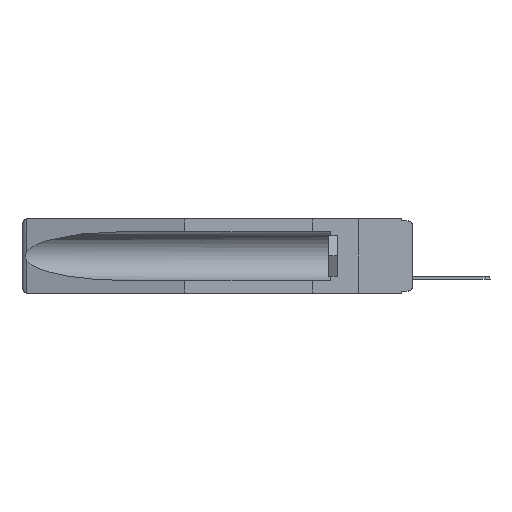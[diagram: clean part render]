
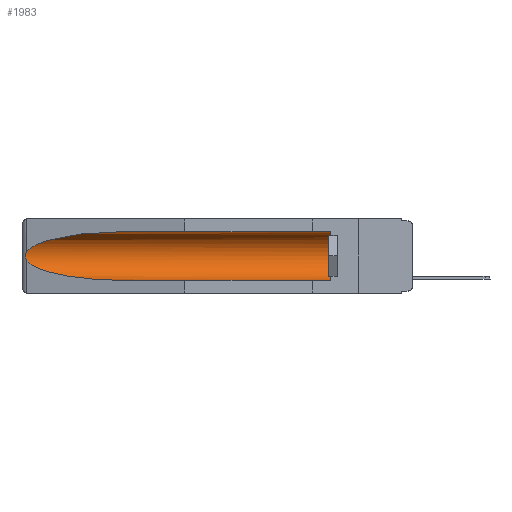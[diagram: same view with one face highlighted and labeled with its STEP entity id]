
A CAD part, left-side view. The second image highlights one B-rep face of the part: STEP entity #1983.
In plain terms, the highlighted cylindrical face has radius 2.857 mm (diameter 5.715 mm), a partial arc.
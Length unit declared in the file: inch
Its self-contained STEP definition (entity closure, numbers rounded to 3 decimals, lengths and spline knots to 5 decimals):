
#101 = CARTESIAN_POINT ( 'NONE',  ( 0.2673, 1.5327, -0.16383 ) ) ;
#332 = EDGE_CURVE ( 'NONE', #722, #12082, #7888, .T. ) ;
#456 = CARTESIAN_POINT ( 'NONE',  ( 0.26537, 1.52718, -0.14972 ) ) ;
#722 = VERTEX_POINT ( 'NONE', #13602 ) ;
#1159 = VECTOR ( 'NONE', #16633, 39.37008 ) ;
#1663 = CARTESIAN_POINT ( 'NONE',  ( 0.2673, 1.53269, -0.17917 ) ) ;
#1698 = LINE ( 'NONE', #4538, #1159 ) ;
#1733 =( BOUNDED_CURVE ( )  B_SPLINE_CURVE ( 3, ( #2733, #14712, #4398, #21807 ),
 .UNSPECIFIED., .F., .T. ) 
 B_SPLINE_CURVE_WITH_KNOTS ( ( 4, 4 ),
 ( 0.1948, 1.5708 ),
 .UNSPECIFIED. ) 
 CURVE ( )  GEOMETRIC_REPRESENTATION_ITEM ( )  RATIONAL_B_SPLINE_CURVE ( ( 1., 0.848, 0.848, 1. ) ) 
 REPRESENTATION_ITEM ( '' )  );
#1983 = ADVANCED_FACE ( 'NONE', ( #13532 ), #9690, .F. ) ;
#2195 = DIRECTION ( 'NONE',  ( 0., 1., 0. ) ) ;
#2305 = DIRECTION ( 'NONE',  ( 0., 0., 1. ) ) ;
#2733 = CARTESIAN_POINT ( 'NONE',  ( 0.26537, 1.52718, -0.19328 ) ) ;
#3238 = CARTESIAN_POINT ( 'NONE',  ( 0.26654, 1.53092, -0.15636 ) ) ;
#3506 = AXIS2_PLACEMENT_3D ( 'NONE', #3848, #2195, #12322 ) ;
#3848 = CARTESIAN_POINT ( 'NONE',  ( 0.155, -0.30754, -0.1715 ) ) ;
#4398 = CARTESIAN_POINT ( 'NONE',  ( 0.21114, 1.30732, -0.284 ) ) ;
#4538 = CARTESIAN_POINT ( 'NONE',  ( 0.155, -0.30754, -0.284 ) ) ;
#4539 = CARTESIAN_POINT ( 'NONE',  ( 0.26537, 1.52718, -0.19328 ) ) ;
#4544 = EDGE_CURVE ( 'NONE', #11175, #722, #14875, .T. ) ;
#4991 = CARTESIAN_POINT ( 'NONE',  ( 0.26597, 1.5296, -0.19026 ) ) ;
#5492 = VECTOR ( 'NONE', #21115, 39.37008 ) ;
#5502 = CARTESIAN_POINT ( 'NONE',  ( 0.155, -0.30754, -0.059 ) ) ;
#6354 = CARTESIAN_POINT ( 'NONE',  ( 0.155, 0.126, -0.059 ) ) ;
#6589 = LINE ( 'NONE', #5502, #5492 ) ;
#6647 = CARTESIAN_POINT ( 'NONE',  ( 0.26537, 1.52718, -0.19328 ) ) ;
#6858 = CARTESIAN_POINT ( 'NONE',  ( 0.2675, 1.53308, -0.16763 ) ) ;
#7267 = DIRECTION ( 'NONE',  ( 0., -1., 0. ) ) ;
#7547 = CIRCLE ( 'NONE', #21148, 0.1125 ) ;
#7888 = B_SPLINE_CURVE_WITH_KNOTS ( 'NONE', 3,
 ( #18815, #17223, #3238, #101, #6858, #8518, #1663, #8581, #4991, #6647 ),
 .UNSPECIFIED., .F., .F.,
 ( 4, 2, 2, 2, 4 ),
 ( 0., 0.00029, 0.00058, 0.00087, 0.00117 ),
 .UNSPECIFIED. ) ;
#8344 = VERTEX_POINT ( 'NONE', #6354 ) ;
#8518 = CARTESIAN_POINT ( 'NONE',  ( 0.2675, 1.53308, -0.17534 ) ) ;
#8581 = CARTESIAN_POINT ( 'NONE',  ( 0.26655, 1.53094, -0.18657 ) ) ;
#9365 = VERTEX_POINT ( 'NONE', #11696 ) ;
#9690 = CYLINDRICAL_SURFACE ( 'NONE', #3506, 0.1125 ) ;
#9703 = VERTEX_POINT ( 'NONE', #16885 ) ;
#10444 = CARTESIAN_POINT ( 'NONE',  ( 0.155, 1.07973, -0.059 ) ) ;
#10650 = EDGE_CURVE ( 'NONE', #8344, #11175, #6589, .T. ) ;
#10750 = CARTESIAN_POINT ( 'NONE',  ( 0.25451, 1.48313, -0.09465 ) ) ;
#11175 = VERTEX_POINT ( 'NONE', #22150 ) ;
#11239 = ORIENTED_EDGE ( 'NONE', *, *, #332, .T. ) ;
#11696 = CARTESIAN_POINT ( 'NONE',  ( 0.155, 1.07973, -0.284 ) ) ;
#12082 = VERTEX_POINT ( 'NONE', #4539 ) ;
#12322 = DIRECTION ( 'NONE',  ( 0., 0., 1. ) ) ;
#13490 = ORIENTED_EDGE ( 'NONE', *, *, #4544, .T. ) ;
#13532 = FACE_OUTER_BOUND ( 'NONE', #21799, .T. ) ;
#13602 = CARTESIAN_POINT ( 'NONE',  ( 0.26537, 1.52718, -0.14972 ) ) ;
#14052 = CARTESIAN_POINT ( 'NONE',  ( 0.21114, 1.30732, -0.059 ) ) ;
#14712 = CARTESIAN_POINT ( 'NONE',  ( 0.25451, 1.48313, -0.24835 ) ) ;
#14875 =( BOUNDED_CURVE ( )  B_SPLINE_CURVE ( 3, ( #10444, #14052, #10750, #456 ),
 .UNSPECIFIED., .F., .F. ) 
 B_SPLINE_CURVE_WITH_KNOTS ( ( 4, 4 ),
 ( 4.71239, 6.08839 ),
 .UNSPECIFIED. ) 
 CURVE ( )  GEOMETRIC_REPRESENTATION_ITEM ( )  RATIONAL_B_SPLINE_CURVE ( ( 1., 0.848, 0.848, 1. ) ) 
 REPRESENTATION_ITEM ( '' )  );
#15667 = EDGE_CURVE ( 'NONE', #12082, #9365, #1733, .T. ) ;
#15736 = EDGE_CURVE ( 'NONE', #9703, #9365, #1698, .T. ) ;
#15853 = ORIENTED_EDGE ( 'NONE', *, *, #15667, .T. ) ;
#16633 = DIRECTION ( 'NONE',  ( 0., 1., 0. ) ) ;
#16885 = CARTESIAN_POINT ( 'NONE',  ( 0.155, 0.126, -0.284 ) ) ;
#17223 = CARTESIAN_POINT ( 'NONE',  ( 0.26597, 1.52961, -0.15275 ) ) ;
#17559 = CARTESIAN_POINT ( 'NONE',  ( 0.155, 0.126, -0.1715 ) ) ;
#17846 = ORIENTED_EDGE ( 'NONE', *, *, #15736, .F. ) ;
#18497 = ORIENTED_EDGE ( 'NONE', *, *, #10650, .T. ) ;
#18815 = CARTESIAN_POINT ( 'NONE',  ( 0.26537, 1.52718, -0.14972 ) ) ;
#20477 = EDGE_CURVE ( 'NONE', #9703, #8344, #7547, .T. ) ;
#21115 = DIRECTION ( 'NONE',  ( 0., 1., 0. ) ) ;
#21148 = AXIS2_PLACEMENT_3D ( 'NONE', #17559, #7267, #2305 ) ;
#21657 = ORIENTED_EDGE ( 'NONE', *, *, #20477, .T. ) ;
#21799 = EDGE_LOOP ( 'NONE', ( #13490, #11239, #15853, #17846, #21657, #18497 ) ) ;
#21807 = CARTESIAN_POINT ( 'NONE',  ( 0.155, 1.07973, -0.284 ) ) ;
#22150 = CARTESIAN_POINT ( 'NONE',  ( 0.155, 1.07973, -0.059 ) ) ;
